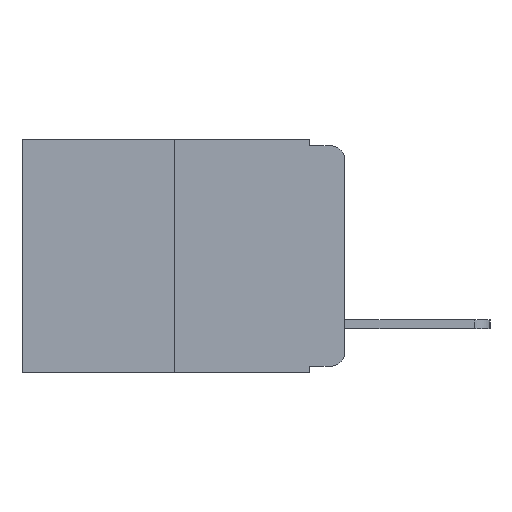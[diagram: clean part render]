
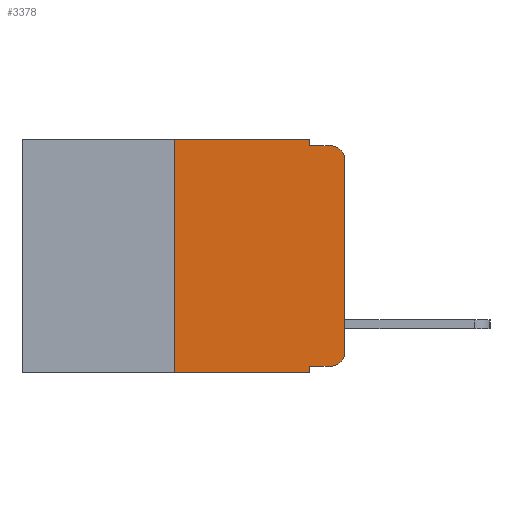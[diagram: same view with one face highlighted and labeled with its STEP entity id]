
A CAD part, left-side view. The second image highlights one B-rep face of the part: STEP entity #3378.
In plain terms, the highlighted planar face has unit normal (-1, 0, 0).
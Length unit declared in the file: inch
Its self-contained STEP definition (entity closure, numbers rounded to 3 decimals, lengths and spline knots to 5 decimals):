
#15 = EDGE_CURVE ( 'NONE', #11794, #4819, #1651, .T. ) ;
#19 = EDGE_CURVE ( 'NONE', #10403, #11794, #1251, .T. ) ;
#21 = DIRECTION ( 'NONE',  ( 0., 0., -1. ) ) ;
#40 = EDGE_CURVE ( 'NONE', #2496, #7371, #10902, .T. ) ;
#105 = EDGE_CURVE ( 'NONE', #9253, #4861, #12382, .T. ) ;
#126 = EDGE_CURVE ( 'NONE', #9253, #3611, #2544, .T. ) ;
#263 = EDGE_CURVE ( 'NONE', #3611, #5848, #6966, .T. ) ;
#280 = DIRECTION ( 'NONE',  ( -1., 0., 0. ) ) ;
#344 = VERTEX_POINT ( 'NONE', #1665 ) ;
#446 = VECTOR ( 'NONE', #12434, 39.37008 ) ;
#863 = CARTESIAN_POINT ( 'NONE',  ( 0., 0.25, -0.343 ) ) ;
#883 = EDGE_CURVE ( 'NONE', #7371, #10403, #5939, .T. ) ;
#1007 = ORIENTED_EDGE ( 'NONE', *, *, #11012, .T. ) ;
#1153 = ORIENTED_EDGE ( 'NONE', *, *, #883, .F. ) ;
#1157 = DIRECTION ( 'NONE',  ( 0., -1., 0. ) ) ;
#1188 = ORIENTED_EDGE ( 'NONE', *, *, #126, .T. ) ;
#1251 = LINE ( 'NONE', #6308, #6549 ) ;
#1323 = PLANE ( 'NONE',  #7306 ) ;
#1354 = CARTESIAN_POINT ( 'NONE',  ( 0., 0.25, 0. ) ) ;
#1375 = CARTESIAN_POINT ( 'NONE',  ( 0., 0.02, -0.01 ) ) ;
#1633 = ORIENTED_EDGE ( 'NONE', *, *, #19, .F. ) ;
#1651 = LINE ( 'NONE', #3338, #11140 ) ;
#1665 = CARTESIAN_POINT ( 'NONE',  ( 0., 0., -0.03 ) ) ;
#2496 = VERTEX_POINT ( 'NONE', #863 ) ;
#2544 = LINE ( 'NONE', #12114, #7549 ) ;
#3338 = CARTESIAN_POINT ( 'NONE',  ( 0., 0.051, -0.01 ) ) ;
#3378 = ADVANCED_FACE ( 'NONE', ( #4954 ), #1323, .F. ) ;
#3466 = AXIS2_PLACEMENT_3D ( 'NONE', #11776, #6577, #21 ) ;
#3611 = VERTEX_POINT ( 'NONE', #9640 ) ;
#3725 = ORIENTED_EDGE ( 'NONE', *, *, #15, .F. ) ;
#3732 = DIRECTION ( 'NONE',  ( 1., 0., 0. ) ) ;
#4688 = CARTESIAN_POINT ( 'NONE',  ( 0., 0.473, 0. ) ) ;
#4804 = LINE ( 'NONE', #11503, #9359 ) ;
#4819 = VERTEX_POINT ( 'NONE', #1375 ) ;
#4861 = VERTEX_POINT ( 'NONE', #8502 ) ;
#4890 = ORIENTED_EDGE ( 'NONE', *, *, #9072, .T. ) ;
#4954 = FACE_OUTER_BOUND ( 'NONE', #5411, .T. ) ;
#5145 = ORIENTED_EDGE ( 'NONE', *, *, #263, .T. ) ;
#5361 = VECTOR ( 'NONE', #8076, 39.37008 ) ;
#5411 = EDGE_LOOP ( 'NONE', ( #5646, #4890, #3725, #1633, #1153, #11548, #1007, #11084, #1188, #5145 ) ) ;
#5646 = ORIENTED_EDGE ( 'NONE', *, *, #12199, .T. ) ;
#5848 = VERTEX_POINT ( 'NONE', #10622 ) ;
#5939 = LINE ( 'NONE', #10041, #10385 ) ;
#6308 = CARTESIAN_POINT ( 'NONE',  ( 0., 0.051, 0. ) ) ;
#6441 = LINE ( 'NONE', #6799, #8559 ) ;
#6549 = VECTOR ( 'NONE', #9863, 39.37008 ) ;
#6577 = DIRECTION ( 'NONE',  ( -1., 0., 0. ) ) ;
#6796 = CARTESIAN_POINT ( 'NONE',  ( 0., 0.051, -0.01 ) ) ;
#6799 = CARTESIAN_POINT ( 'NONE',  ( 0., 0.473, -0.343 ) ) ;
#6966 = CIRCLE ( 'NONE', #7639, 0.02 ) ;
#7306 = AXIS2_PLACEMENT_3D ( 'NONE', #4688, #3732, #10133 ) ;
#7371 = VERTEX_POINT ( 'NONE', #1354 ) ;
#7549 = VECTOR ( 'NONE', #11214, 39.37008 ) ;
#7639 = AXIS2_PLACEMENT_3D ( 'NONE', #9336, #280, #7679 ) ;
#7679 = DIRECTION ( 'NONE',  ( 0., 0., -1. ) ) ;
#8076 = DIRECTION ( 'NONE',  ( 0., 0., -1. ) ) ;
#8144 = DIRECTION ( 'NONE',  ( 0., 0., 1. ) ) ;
#8502 = CARTESIAN_POINT ( 'NONE',  ( 0., 0.051, -0.343 ) ) ;
#8559 = VECTOR ( 'NONE', #11091, 39.37008 ) ;
#8949 = CARTESIAN_POINT ( 'NONE',  ( 0., 0.051, 0. ) ) ;
#9068 = CARTESIAN_POINT ( 'NONE',  ( 0., 0.25, 0. ) ) ;
#9072 = EDGE_CURVE ( 'NONE', #344, #4819, #9804, .T. ) ;
#9253 = VERTEX_POINT ( 'NONE', #11893 ) ;
#9336 = CARTESIAN_POINT ( 'NONE',  ( 0., 0.02, -0.313 ) ) ;
#9359 = VECTOR ( 'NONE', #8144, 39.37008 ) ;
#9640 = CARTESIAN_POINT ( 'NONE',  ( 0., 0.02, -0.333 ) ) ;
#9804 = CIRCLE ( 'NONE', #3466, 0.02 ) ;
#9863 = DIRECTION ( 'NONE',  ( 0., 0., -1. ) ) ;
#10041 = CARTESIAN_POINT ( 'NONE',  ( 0., 0.473, 0. ) ) ;
#10133 = DIRECTION ( 'NONE',  ( 0., 0., -1. ) ) ;
#10385 = VECTOR ( 'NONE', #1157, 39.37008 ) ;
#10403 = VERTEX_POINT ( 'NONE', #11835 ) ;
#10622 = CARTESIAN_POINT ( 'NONE',  ( 0., 0., -0.313 ) ) ;
#10902 = LINE ( 'NONE', #9068, #446 ) ;
#11012 = EDGE_CURVE ( 'NONE', #2496, #4861, #6441, .T. ) ;
#11084 = ORIENTED_EDGE ( 'NONE', *, *, #105, .F. ) ;
#11091 = DIRECTION ( 'NONE',  ( 0., -1., 0. ) ) ;
#11140 = VECTOR ( 'NONE', #12401, 39.37008 ) ;
#11214 = DIRECTION ( 'NONE',  ( 0., -1., 0. ) ) ;
#11503 = CARTESIAN_POINT ( 'NONE',  ( 0., 0., 0. ) ) ;
#11548 = ORIENTED_EDGE ( 'NONE', *, *, #40, .F. ) ;
#11776 = CARTESIAN_POINT ( 'NONE',  ( 0., 0.02, -0.03 ) ) ;
#11794 = VERTEX_POINT ( 'NONE', #6796 ) ;
#11835 = CARTESIAN_POINT ( 'NONE',  ( 0., 0.051, 0. ) ) ;
#11893 = CARTESIAN_POINT ( 'NONE',  ( 0., 0.051, -0.333 ) ) ;
#12114 = CARTESIAN_POINT ( 'NONE',  ( 0., 0.051, -0.333 ) ) ;
#12199 = EDGE_CURVE ( 'NONE', #5848, #344, #4804, .T. ) ;
#12382 = LINE ( 'NONE', #8949, #5361 ) ;
#12401 = DIRECTION ( 'NONE',  ( 0., -1., 0. ) ) ;
#12434 = DIRECTION ( 'NONE',  ( 0., 0., 1. ) ) ;
